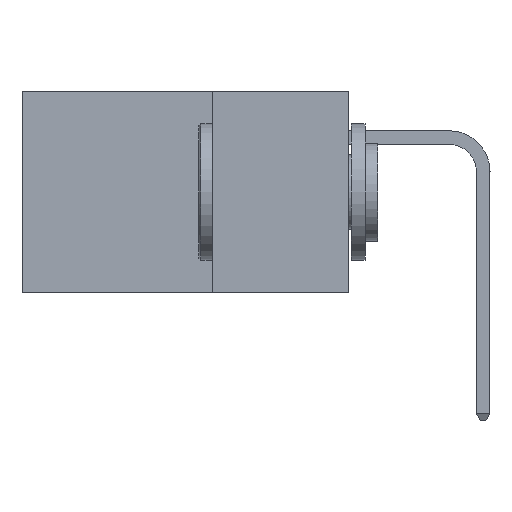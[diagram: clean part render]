
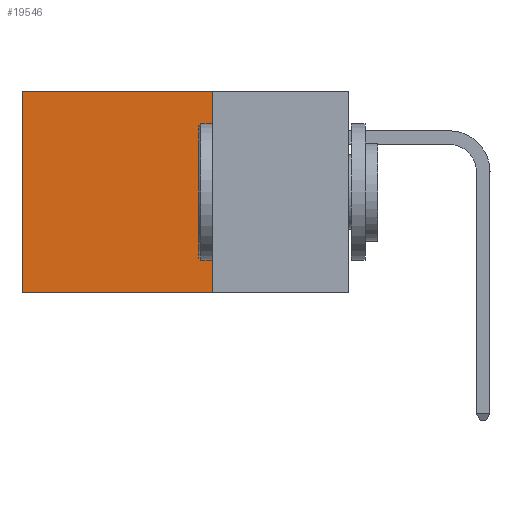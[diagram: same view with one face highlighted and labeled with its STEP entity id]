
A CAD part, left-side view. The second image highlights one B-rep face of the part: STEP entity #19546.
In plain terms, the highlighted planar face has unit normal (-1, 0, 0).
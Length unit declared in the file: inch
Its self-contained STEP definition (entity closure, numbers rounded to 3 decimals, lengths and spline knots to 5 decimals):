
#427 = ORIENTED_EDGE ( 'NONE', *, *, #15863, .T. ) ;
#1941 = CARTESIAN_POINT ( 'NONE',  ( 0.2875, 0.25, 0. ) ) ;
#2198 = DIRECTION ( 'NONE',  ( 0., 0., -1. ) ) ;
#4351 = VERTEX_POINT ( 'NONE', #42592 ) ;
#6775 = DIRECTION ( 'NONE',  ( 1., 0., 0. ) ) ;
#8815 = VERTEX_POINT ( 'NONE', #16424 ) ;
#12516 = CARTESIAN_POINT ( 'NONE',  ( 0.2875, 0.25, -0.37 ) ) ;
#13591 = CARTESIAN_POINT ( 'NONE',  ( 0.2875, 0.25, -0.37 ) ) ;
#14343 = LINE ( 'NONE', #27599, #32800 ) ;
#14461 = VECTOR ( 'NONE', #31947, 39.37008 ) ;
#14465 = ORIENTED_EDGE ( 'NONE', *, *, #18673, .F. ) ;
#15488 = FACE_OUTER_BOUND ( 'NONE', #19184, .T. ) ;
#15863 = EDGE_CURVE ( 'NONE', #29641, #4351, #14343, .T. ) ;
#16424 = CARTESIAN_POINT ( 'NONE',  ( 0.2875, 0.25, 0. ) ) ;
#17062 = CARTESIAN_POINT ( 'NONE',  ( 0.2875, 0.25, 0. ) ) ;
#17598 = EDGE_CURVE ( 'NONE', #8815, #29641, #44684, .T. ) ;
#18673 = EDGE_CURVE ( 'NONE', #21160, #4351, #45776, .T. ) ;
#19184 = EDGE_LOOP ( 'NONE', ( #427, #14465, #28903, #28769 ) ) ;
#19240 = CARTESIAN_POINT ( 'NONE',  ( 0.2875, 0.6, 0. ) ) ;
#19546 = ADVANCED_FACE ( 'NONE', ( #15488 ), #21202, .F. ) ;
#20370 = EDGE_CURVE ( 'NONE', #8815, #21160, #26309, .T. ) ;
#21160 = VERTEX_POINT ( 'NONE', #13591 ) ;
#21202 = PLANE ( 'NONE',  #36220 ) ;
#23399 = DIRECTION ( 'NONE',  ( 0., 1., 0. ) ) ;
#24935 = CARTESIAN_POINT ( 'NONE',  ( 0.2875, 0.25, 0. ) ) ;
#26309 = LINE ( 'NONE', #1941, #45607 ) ;
#27509 = DIRECTION ( 'NONE',  ( 0., 0., -1. ) ) ;
#27599 = CARTESIAN_POINT ( 'NONE',  ( 0.2875, 0.6, 0. ) ) ;
#28769 = ORIENTED_EDGE ( 'NONE', *, *, #17598, .T. ) ;
#28903 = ORIENTED_EDGE ( 'NONE', *, *, #20370, .F. ) ;
#29641 = VERTEX_POINT ( 'NONE', #19240 ) ;
#31947 = DIRECTION ( 'NONE',  ( 0., 1., 0. ) ) ;
#32427 = DIRECTION ( 'NONE',  ( 0., 0., -1. ) ) ;
#32800 = VECTOR ( 'NONE', #2198, 39.37008 ) ;
#36220 = AXIS2_PLACEMENT_3D ( 'NONE', #24935, #6775, #32427 ) ;
#42592 = CARTESIAN_POINT ( 'NONE',  ( 0.2875, 0.6, -0.37 ) ) ;
#44646 = VECTOR ( 'NONE', #23399, 39.37008 ) ;
#44684 = LINE ( 'NONE', #17062, #14461 ) ;
#45607 = VECTOR ( 'NONE', #27509, 39.37008 ) ;
#45776 = LINE ( 'NONE', #12516, #44646 ) ;
